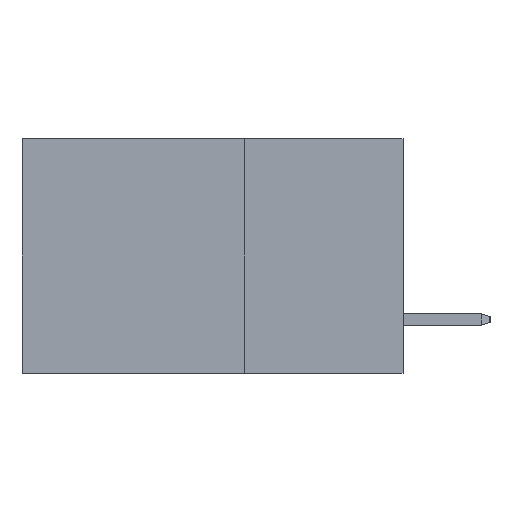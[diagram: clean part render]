
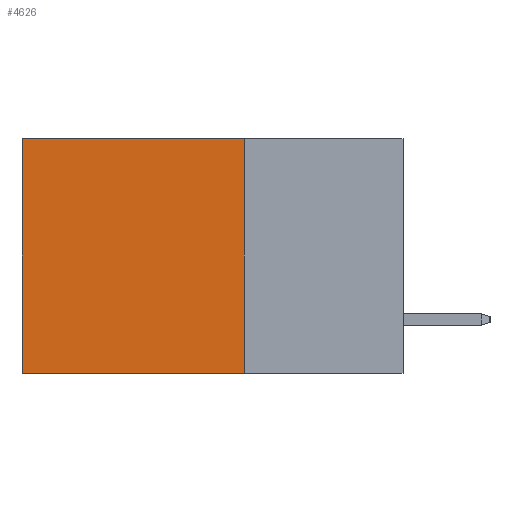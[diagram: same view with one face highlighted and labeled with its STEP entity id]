
A CAD part, left-side view. The second image highlights one B-rep face of the part: STEP entity #4626.
In plain terms, the highlighted planar face has unit normal (-1, 0, 0).
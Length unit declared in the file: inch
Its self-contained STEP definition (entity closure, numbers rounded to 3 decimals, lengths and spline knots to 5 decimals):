
#206 = EDGE_CURVE ( 'NONE', #10523, #9904, #5167, .T. ) ;
#651 = EDGE_LOOP ( 'NONE', ( #8799, #7266, #4044, #7362 ) ) ;
#775 = AXIS2_PLACEMENT_3D ( 'NONE', #8488, #5707, #1300 ) ;
#1300 = DIRECTION ( 'NONE',  ( 0., 0., -1. ) ) ;
#1448 = LINE ( 'NONE', #4938, #4409 ) ;
#1483 = FACE_OUTER_BOUND ( 'NONE', #651, .T. ) ;
#1674 = DIRECTION ( 'NONE',  ( 0., 0., -1. ) ) ;
#1719 = CARTESIAN_POINT ( 'NONE',  ( 0.2875, 0.25, 0. ) ) ;
#3143 = VECTOR ( 'NONE', #4196, 39.37008 ) ;
#3386 = CARTESIAN_POINT ( 'NONE',  ( 0.2875, 0.6, 0. ) ) ;
#3498 = EDGE_CURVE ( 'NONE', #10523, #10346, #1448, .T. ) ;
#3723 = DIRECTION ( 'NONE',  ( 0., 1., 0. ) ) ;
#4044 = ORIENTED_EDGE ( 'NONE', *, *, #206, .F. ) ;
#4196 = DIRECTION ( 'NONE',  ( 0., 0., -1. ) ) ;
#4409 = VECTOR ( 'NONE', #6550, 39.37008 ) ;
#4626 = ADVANCED_FACE ( 'NONE', ( #1483 ), #5646, .F. ) ;
#4818 = CARTESIAN_POINT ( 'NONE',  ( 0.2875, 0.6, -0.37 ) ) ;
#4938 = CARTESIAN_POINT ( 'NONE',  ( 0.2875, 0.25, 0. ) ) ;
#5167 = LINE ( 'NONE', #6717, #3143 ) ;
#5646 = PLANE ( 'NONE',  #775 ) ;
#5707 = DIRECTION ( 'NONE',  ( 1., 0., 0. ) ) ;
#6021 = LINE ( 'NONE', #9534, #7177 ) ;
#6531 = CARTESIAN_POINT ( 'NONE',  ( 0.2875, 0.25, -0.37 ) ) ;
#6550 = DIRECTION ( 'NONE',  ( 0., 1., 0. ) ) ;
#6709 = EDGE_CURVE ( 'NONE', #9904, #8623, #8083, .T. ) ;
#6717 = CARTESIAN_POINT ( 'NONE',  ( 0.2875, 0.25, 0. ) ) ;
#7045 = CARTESIAN_POINT ( 'NONE',  ( 0.2875, 0.25, -0.37 ) ) ;
#7177 = VECTOR ( 'NONE', #1674, 39.37008 ) ;
#7215 = EDGE_CURVE ( 'NONE', #10346, #8623, #6021, .T. ) ;
#7266 = ORIENTED_EDGE ( 'NONE', *, *, #6709, .F. ) ;
#7362 = ORIENTED_EDGE ( 'NONE', *, *, #3498, .T. ) ;
#8083 = LINE ( 'NONE', #7045, #8825 ) ;
#8488 = CARTESIAN_POINT ( 'NONE',  ( 0.2875, 0.25, 0. ) ) ;
#8623 = VERTEX_POINT ( 'NONE', #4818 ) ;
#8799 = ORIENTED_EDGE ( 'NONE', *, *, #7215, .T. ) ;
#8825 = VECTOR ( 'NONE', #3723, 39.37008 ) ;
#9534 = CARTESIAN_POINT ( 'NONE',  ( 0.2875, 0.6, 0. ) ) ;
#9904 = VERTEX_POINT ( 'NONE', #6531 ) ;
#10346 = VERTEX_POINT ( 'NONE', #3386 ) ;
#10523 = VERTEX_POINT ( 'NONE', #1719 ) ;
